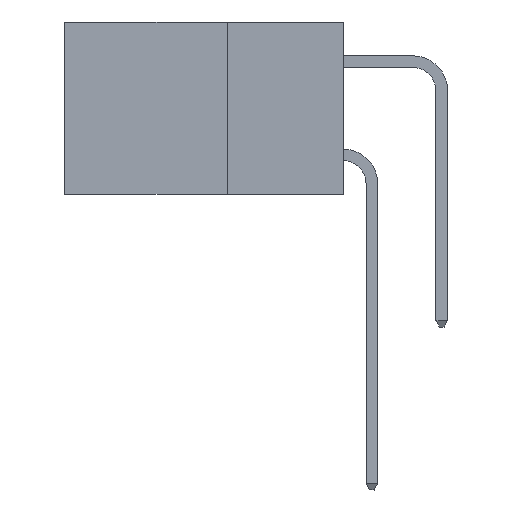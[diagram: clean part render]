
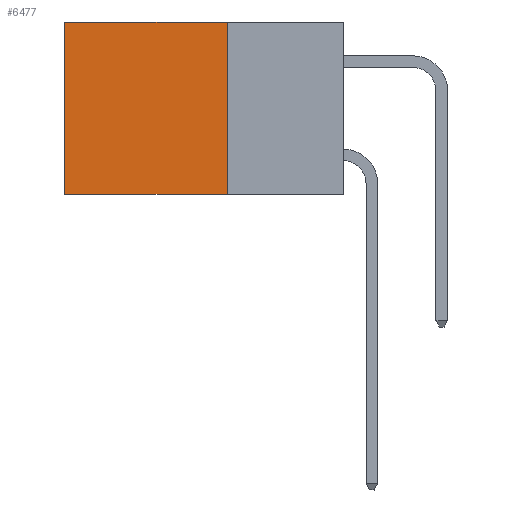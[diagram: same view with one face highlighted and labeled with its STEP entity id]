
A CAD part, left-side view. The second image highlights one B-rep face of the part: STEP entity #6477.
In plain terms, the highlighted planar face has unit normal (-1, 0, 0).
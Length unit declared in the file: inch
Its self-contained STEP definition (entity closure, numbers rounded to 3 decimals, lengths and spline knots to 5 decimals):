
#287 = DIRECTION ( 'NONE',  ( 1., 0., 0. ) ) ;
#534 = LINE ( 'NONE', #6942, #986 ) ;
#592 = VECTOR ( 'NONE', #2814, 39.37008 ) ;
#652 = CARTESIAN_POINT ( 'NONE',  ( 0.2615, 0.25, -0.37 ) ) ;
#817 = VECTOR ( 'NONE', #1832, 39.37008 ) ;
#860 = CARTESIAN_POINT ( 'NONE',  ( 0.2615, 0.6, -0.37 ) ) ;
#986 = VECTOR ( 'NONE', #2172, 39.37008 ) ;
#1832 = DIRECTION ( 'NONE',  ( 0., 0., -1. ) ) ;
#1901 = VECTOR ( 'NONE', #3874, 39.37008 ) ;
#2097 = CARTESIAN_POINT ( 'NONE',  ( 0.2615, 0.25, 0. ) ) ;
#2172 = DIRECTION ( 'NONE',  ( 0., 0., -1. ) ) ;
#2701 = EDGE_LOOP ( 'NONE', ( #8220, #4984, #8827, #5462 ) ) ;
#2814 = DIRECTION ( 'NONE',  ( 0., 1., 0. ) ) ;
#3109 = VERTEX_POINT ( 'NONE', #5218 ) ;
#3447 = CARTESIAN_POINT ( 'NONE',  ( 0.2615, 0.25, 0. ) ) ;
#3602 = VERTEX_POINT ( 'NONE', #3447 ) ;
#3743 = CARTESIAN_POINT ( 'NONE',  ( 0.2615, 0.6, -0.37 ) ) ;
#3874 = DIRECTION ( 'NONE',  ( 0., 1., 0. ) ) ;
#4035 = EDGE_CURVE ( 'NONE', #3109, #8536, #6444, .T. ) ;
#4694 = VERTEX_POINT ( 'NONE', #4983 ) ;
#4983 = CARTESIAN_POINT ( 'NONE',  ( 0.2615, 0.6, 0. ) ) ;
#4984 = ORIENTED_EDGE ( 'NONE', *, *, #4035, .F. ) ;
#4998 = CARTESIAN_POINT ( 'NONE',  ( 0.2615, 0.25, -0.37 ) ) ;
#5049 = FACE_OUTER_BOUND ( 'NONE', #2701, .T. ) ;
#5218 = CARTESIAN_POINT ( 'NONE',  ( 0.2615, 0.25, -0.37 ) ) ;
#5462 = ORIENTED_EDGE ( 'NONE', *, *, #7668, .T. ) ;
#6444 = LINE ( 'NONE', #652, #1901 ) ;
#6477 = ADVANCED_FACE ( 'NONE', ( #5049 ), #6662, .F. ) ;
#6662 = PLANE ( 'NONE',  #8649 ) ;
#6942 = CARTESIAN_POINT ( 'NONE',  ( 0.2615, 0.25, -0.37 ) ) ;
#7668 = EDGE_CURVE ( 'NONE', #3602, #4694, #9257, .T. ) ;
#8169 = LINE ( 'NONE', #860, #817 ) ;
#8190 = DIRECTION ( 'NONE',  ( 0., 0., -1. ) ) ;
#8220 = ORIENTED_EDGE ( 'NONE', *, *, #10159, .T. ) ;
#8536 = VERTEX_POINT ( 'NONE', #3743 ) ;
#8649 = AXIS2_PLACEMENT_3D ( 'NONE', #4998, #287, #8190 ) ;
#8827 = ORIENTED_EDGE ( 'NONE', *, *, #10096, .F. ) ;
#9257 = LINE ( 'NONE', #2097, #592 ) ;
#10096 = EDGE_CURVE ( 'NONE', #3602, #3109, #534, .T. ) ;
#10159 = EDGE_CURVE ( 'NONE', #4694, #8536, #8169, .T. ) ;
